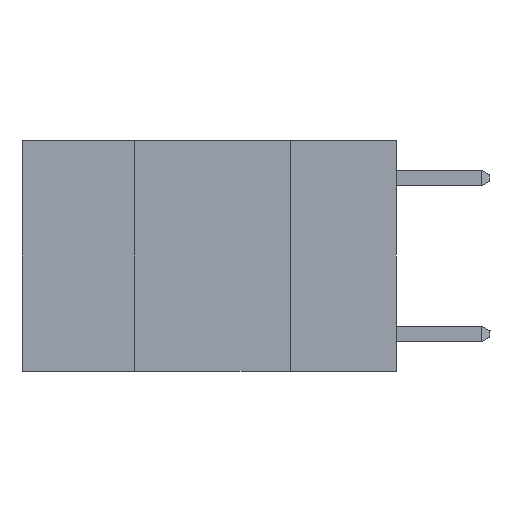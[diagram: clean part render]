
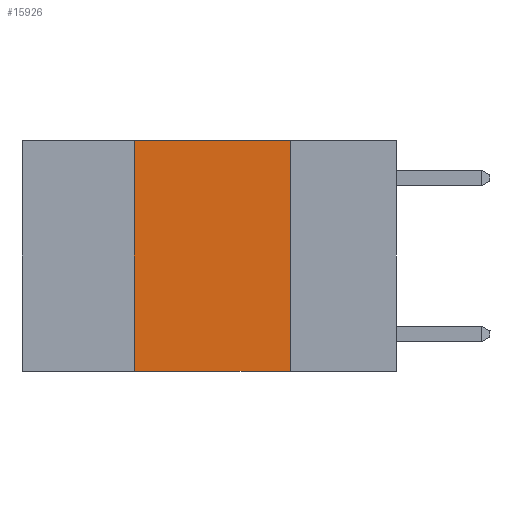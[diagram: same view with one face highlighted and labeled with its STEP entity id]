
A CAD part, left-side view. The second image highlights one B-rep face of the part: STEP entity #15926.
In plain terms, the highlighted planar face has unit normal (-1, 0, 0).
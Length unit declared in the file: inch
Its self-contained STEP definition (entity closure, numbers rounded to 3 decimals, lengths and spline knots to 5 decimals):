
#1143 = EDGE_CURVE ( 'NONE', #26893, #17816, #9595, .T. ) ;
#1385 = LINE ( 'NONE', #15829, #11779 ) ;
#1919 = CARTESIAN_POINT ( 'NONE',  ( 0., 0.42, 0. ) ) ;
#2082 = DIRECTION ( 'NONE',  ( 1., 0., 0. ) ) ;
#2216 = ORIENTED_EDGE ( 'NONE', *, *, #22868, .F. ) ;
#3839 = CARTESIAN_POINT ( 'NONE',  ( 0., 0.17, 0. ) ) ;
#4463 = VECTOR ( 'NONE', #18977, 39.37008 ) ;
#5625 = FACE_OUTER_BOUND ( 'NONE', #11504, .T. ) ;
#5851 = ORIENTED_EDGE ( 'NONE', *, *, #21142, .F. ) ;
#6794 = PLANE ( 'NONE',  #14523 ) ;
#7298 = CARTESIAN_POINT ( 'NONE',  ( 0., 0.6, -0.37 ) ) ;
#8624 = DIRECTION ( 'NONE',  ( 0., 0., -1. ) ) ;
#9583 = CARTESIAN_POINT ( 'NONE',  ( 0., 0.42, 0. ) ) ;
#9587 = VECTOR ( 'NONE', #18980, 39.37008 ) ;
#9595 = LINE ( 'NONE', #7298, #9587 ) ;
#9934 = VERTEX_POINT ( 'NONE', #1919 ) ;
#10895 = VECTOR ( 'NONE', #8624, 39.37008 ) ;
#11286 = DIRECTION ( 'NONE',  ( 0., -1., 0. ) ) ;
#11295 = EDGE_CURVE ( 'NONE', #9934, #27041, #1385, .T. ) ;
#11504 = EDGE_LOOP ( 'NONE', ( #5851, #13583, #2216, #12470 ) ) ;
#11779 = VECTOR ( 'NONE', #11286, 39.37008 ) ;
#12470 = ORIENTED_EDGE ( 'NONE', *, *, #1143, .T. ) ;
#13583 = ORIENTED_EDGE ( 'NONE', *, *, #11295, .F. ) ;
#14523 = AXIS2_PLACEMENT_3D ( 'NONE', #27785, #2082, #18541 ) ;
#15614 = CARTESIAN_POINT ( 'NONE',  ( 0., 0.17, 0. ) ) ;
#15829 = CARTESIAN_POINT ( 'NONE',  ( 0., 0.6, 0. ) ) ;
#15926 = ADVANCED_FACE ( 'NONE', ( #5625 ), #6794, .F. ) ;
#17816 = VERTEX_POINT ( 'NONE', #29803 ) ;
#18541 = DIRECTION ( 'NONE',  ( 0., 0., -1. ) ) ;
#18977 = DIRECTION ( 'NONE',  ( 0., 0., 1. ) ) ;
#18980 = DIRECTION ( 'NONE',  ( 0., -1., 0. ) ) ;
#21142 = EDGE_CURVE ( 'NONE', #27041, #17816, #22599, .T. ) ;
#22599 = LINE ( 'NONE', #3839, #10895 ) ;
#22868 = EDGE_CURVE ( 'NONE', #26893, #9934, #27874, .T. ) ;
#24477 = CARTESIAN_POINT ( 'NONE',  ( 0., 0.42, -0.37 ) ) ;
#26893 = VERTEX_POINT ( 'NONE', #24477 ) ;
#27041 = VERTEX_POINT ( 'NONE', #15614 ) ;
#27785 = CARTESIAN_POINT ( 'NONE',  ( 0., 0.6, 0. ) ) ;
#27874 = LINE ( 'NONE', #9583, #4463 ) ;
#29803 = CARTESIAN_POINT ( 'NONE',  ( 0., 0.17, -0.37 ) ) ;
